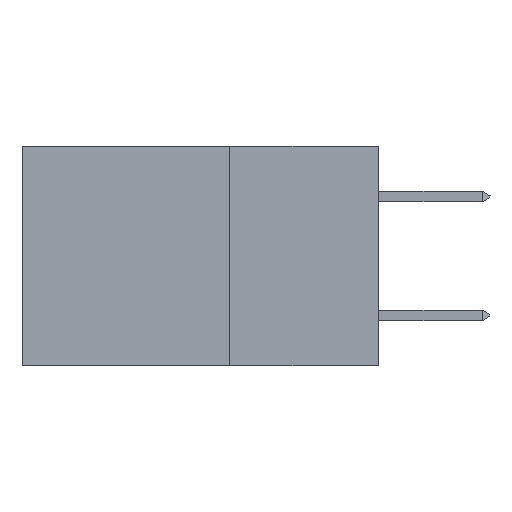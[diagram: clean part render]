
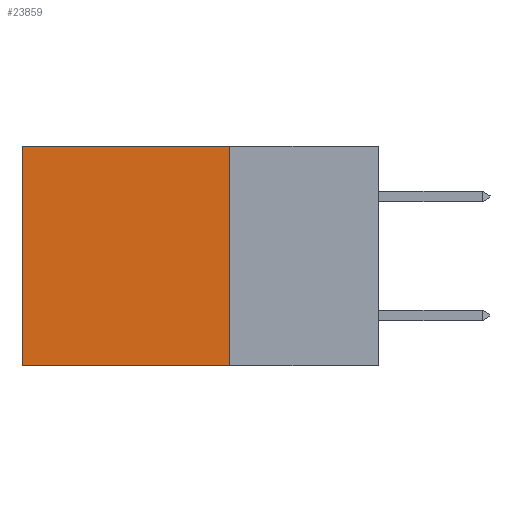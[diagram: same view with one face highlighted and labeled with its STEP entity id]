
A CAD part, left-side view. The second image highlights one B-rep face of the part: STEP entity #23859.
In plain terms, the highlighted planar face has unit normal (-1, 0, 0).
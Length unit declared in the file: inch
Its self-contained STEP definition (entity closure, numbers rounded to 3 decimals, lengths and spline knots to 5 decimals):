
#219 = ORIENTED_EDGE ( 'NONE', *, *, #11232, .F. ) ;
#789 = CARTESIAN_POINT ( 'NONE',  ( 0.2615, 0.25, -0.37 ) ) ;
#979 = DIRECTION ( 'NONE',  ( 1., 0., 0. ) ) ;
#1596 = CARTESIAN_POINT ( 'NONE',  ( 0.2615, 0.25, -0.37 ) ) ;
#2812 = AXIS2_PLACEMENT_3D ( 'NONE', #13893, #979, #19395 ) ;
#3786 = CARTESIAN_POINT ( 'NONE',  ( 0.2615, 0.25, 0. ) ) ;
#3808 = CARTESIAN_POINT ( 'NONE',  ( 0.2615, 0.6, -0.37 ) ) ;
#3842 = DIRECTION ( 'NONE',  ( 0., 1., 0. ) ) ;
#4110 = LINE ( 'NONE', #789, #17352 ) ;
#4995 = DIRECTION ( 'NONE',  ( 0., 1., 0. ) ) ;
#6222 = VECTOR ( 'NONE', #3842, 39.37008 ) ;
#6565 = PLANE ( 'NONE',  #2812 ) ;
#6776 = EDGE_LOOP ( 'NONE', ( #15941, #219, #11043, #8863 ) ) ;
#7112 = CARTESIAN_POINT ( 'NONE',  ( 0.2615, 0.6, 0. ) ) ;
#7986 = DIRECTION ( 'NONE',  ( 0., 0., -1. ) ) ;
#8863 = ORIENTED_EDGE ( 'NONE', *, *, #16559, .T. ) ;
#9242 = CARTESIAN_POINT ( 'NONE',  ( 0.2615, 0.6, -0.37 ) ) ;
#11043 = ORIENTED_EDGE ( 'NONE', *, *, #19594, .F. ) ;
#11232 = EDGE_CURVE ( 'NONE', #13376, #20244, #18230, .T. ) ;
#11662 = VERTEX_POINT ( 'NONE', #3786 ) ;
#12673 = LINE ( 'NONE', #9242, #13766 ) ;
#13376 = VERTEX_POINT ( 'NONE', #1596 ) ;
#13766 = VECTOR ( 'NONE', #16695, 39.37008 ) ;
#13893 = CARTESIAN_POINT ( 'NONE',  ( 0.2615, 0.25, -0.37 ) ) ;
#15568 = EDGE_CURVE ( 'NONE', #23216, #20244, #12673, .T. ) ;
#15744 = FACE_OUTER_BOUND ( 'NONE', #6776, .T. ) ;
#15941 = ORIENTED_EDGE ( 'NONE', *, *, #15568, .T. ) ;
#15978 = CARTESIAN_POINT ( 'NONE',  ( 0.2615, 0.25, 0. ) ) ;
#16559 = EDGE_CURVE ( 'NONE', #11662, #23216, #21709, .T. ) ;
#16695 = DIRECTION ( 'NONE',  ( 0., 0., -1. ) ) ;
#16838 = VECTOR ( 'NONE', #4995, 39.37008 ) ;
#17352 = VECTOR ( 'NONE', #7986, 39.37008 ) ;
#18230 = LINE ( 'NONE', #23973, #6222 ) ;
#19395 = DIRECTION ( 'NONE',  ( 0., 0., -1. ) ) ;
#19594 = EDGE_CURVE ( 'NONE', #11662, #13376, #4110, .T. ) ;
#20244 = VERTEX_POINT ( 'NONE', #3808 ) ;
#21709 = LINE ( 'NONE', #15978, #16838 ) ;
#23216 = VERTEX_POINT ( 'NONE', #7112 ) ;
#23859 = ADVANCED_FACE ( 'NONE', ( #15744 ), #6565, .F. ) ;
#23973 = CARTESIAN_POINT ( 'NONE',  ( 0.2615, 0.25, -0.37 ) ) ;
